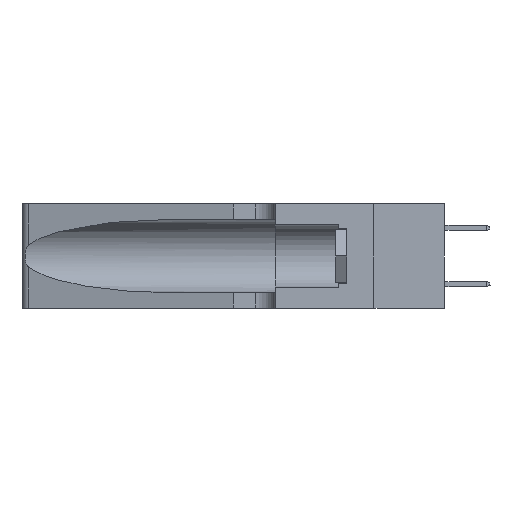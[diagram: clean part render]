
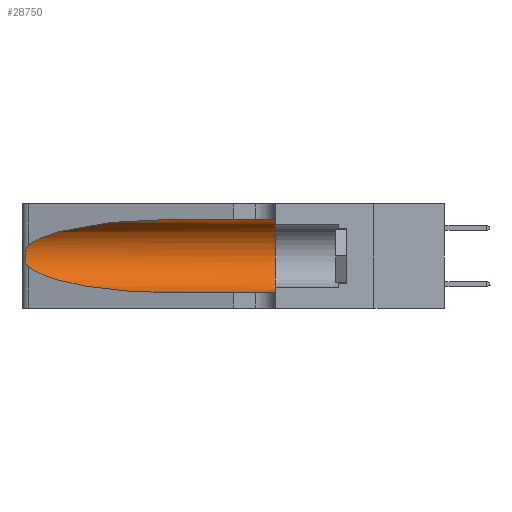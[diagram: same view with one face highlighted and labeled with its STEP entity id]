
A CAD part, left-side view. The second image highlights one B-rep face of the part: STEP entity #28750.
In plain terms, the highlighted cylindrical face has radius 3.308 mm (diameter 6.617 mm), a partial arc.
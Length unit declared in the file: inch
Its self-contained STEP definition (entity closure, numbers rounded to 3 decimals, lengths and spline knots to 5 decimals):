
#1420 = CARTESIAN_POINT ( 'NONE',  ( 0.1305, 0.72297, 0.05475 ) ) ;
#2338 = EDGE_CURVE ( 'NONE', #28870, #16854, #35391, .T. ) ;
#2971 = CARTESIAN_POINT ( 'NONE',  ( 0.25487, 1.22718, 0.14631 ) ) ;
#4224 = EDGE_CURVE ( 'NONE', #25552, #4674, #34730, .T. ) ;
#4225 = AXIS2_PLACEMENT_3D ( 'NONE', #11560, #11099, #27689 ) ;
#4227 = DIRECTION ( 'NONE',  ( 0., 1., 0. ) ) ;
#4668 = ORIENTED_EDGE ( 'NONE', *, *, #24497, .F. ) ;
#4674 = VERTEX_POINT ( 'NONE', #14045 ) ;
#5128 = CARTESIAN_POINT ( 'NONE',  ( 0.1305, 0.72297, 0.05475 ) ) ;
#5406 = EDGE_CURVE ( 'NONE', #4674, #28870, #21373, .T. ) ;
#5975 = CARTESIAN_POINT ( 'NONE',  ( 0.25639, 1.23184, 0.21858 ) ) ;
#7734 = CARTESIAN_POINT ( 'NONE',  ( 0.25487, 1.22718, 0.14631 ) ) ;
#9146 = CARTESIAN_POINT ( 'NONE',  ( 0.25639, 1.23186, 0.15144 ) ) ;
#9158 = EDGE_LOOP ( 'NONE', ( #30131, #21427, #10107, #10745, #4668, #17406 ) ) ;
#9277 = CARTESIAN_POINT ( 'NONE',  ( 0.25854, 1.2359, 0.20912 ) ) ;
#9411 = CARTESIAN_POINT ( 'NONE',  ( 0.25555, 1.22993, 0.14849 ) ) ;
#10107 = ORIENTED_EDGE ( 'NONE', *, *, #5406, .T. ) ;
#10640 = CARTESIAN_POINT ( 'NONE',  ( 0.1305, 0.72297, 0.31525 ) ) ;
#10745 = ORIENTED_EDGE ( 'NONE', *, *, #2338, .T. ) ;
#11099 = DIRECTION ( 'NONE',  ( 0., -1., 0. ) ) ;
#11136 = EDGE_CURVE ( 'NONE', #39856, #25552, #27072, .T. ) ;
#11274 = CARTESIAN_POINT ( 'NONE',  ( 0.2373, 1.15595, 0.28018 ) ) ;
#11437 = VERTEX_POINT ( 'NONE', #25014 ) ;
#11560 = CARTESIAN_POINT ( 'NONE',  ( 0.1305, 1.61858, 0.185 ) ) ;
#11943 = CARTESIAN_POINT ( 'NONE',  ( 0.1305, 0.35, 0.05475 ) ) ;
#12255 = CARTESIAN_POINT ( 'NONE',  ( 0.25787, 1.23484, 0.2124 ) ) ;
#12767 = DIRECTION ( 'NONE',  ( 0., -1., 0. ) ) ;
#14045 = CARTESIAN_POINT ( 'NONE',  ( 0.25487, 1.22718, 0.14631 ) ) ;
#14901 = CARTESIAN_POINT ( 'NONE',  ( 0.25487, 1.22718, 0.22369 ) ) ;
#16854 = VERTEX_POINT ( 'NONE', #11943 ) ;
#17406 = ORIENTED_EDGE ( 'NONE', *, *, #21244, .F. ) ;
#18690 = CARTESIAN_POINT ( 'NONE',  ( 0.25856, 1.23593, 0.16098 ) ) ;
#19502 = VECTOR ( 'NONE', #21400, 39.37008 ) ;
#20017 = CIRCLE ( 'NONE', #24137, 0.13025 ) ;
#20641 = DIRECTION ( 'NONE',  ( 0., 0., 1. ) ) ;
#21244 = EDGE_CURVE ( 'NONE', #39856, #11437, #21584, .T. ) ;
#21373 =( BOUNDED_CURVE ( )  B_SPLINE_CURVE ( 3, ( #7734, #23557, #28028, #1420 ),
 .UNSPECIFIED., .F., .F. ) 
 B_SPLINE_CURVE_WITH_KNOTS ( ( 4, 4 ),
 ( 3.44316, 4.71239 ),
 .UNSPECIFIED. ) 
 CURVE ( )  GEOMETRIC_REPRESENTATION_ITEM ( )  RATIONAL_B_SPLINE_CURVE ( ( 1., 0.87, 0.87, 1. ) ) 
 REPRESENTATION_ITEM ( '' )  );
#21400 = DIRECTION ( 'NONE',  ( 0., -1., 0. ) ) ;
#21427 = ORIENTED_EDGE ( 'NONE', *, *, #4224, .T. ) ;
#21584 = LINE ( 'NONE', #27388, #19502 ) ;
#22190 = FACE_OUTER_BOUND ( 'NONE', #9158, .T. ) ;
#22271 = CARTESIAN_POINT ( 'NONE',  ( 0.25789, 1.23486, 0.15765 ) ) ;
#22523 = CARTESIAN_POINT ( 'NONE',  ( 0.26017, 1.23833, 0.17102 ) ) ;
#23557 = CARTESIAN_POINT ( 'NONE',  ( 0.2373, 1.15595, 0.08982 ) ) ;
#24137 = AXIS2_PLACEMENT_3D ( 'NONE', #40005, #4227, #20641 ) ;
#24497 = EDGE_CURVE ( 'NONE', #11437, #16854, #20017, .T. ) ;
#25014 = CARTESIAN_POINT ( 'NONE',  ( 0.1305, 0.35, 0.31525 ) ) ;
#25552 = VERTEX_POINT ( 'NONE', #14901 ) ;
#27072 =( BOUNDED_CURVE ( )  B_SPLINE_CURVE ( 3, ( #41065, #27386, #11274, #40479 ),
 .UNSPECIFIED., .F., .T. ) 
 B_SPLINE_CURVE_WITH_KNOTS ( ( 4, 4 ),
 ( 1.5708, 2.84003 ),
 .UNSPECIFIED. ) 
 CURVE ( )  GEOMETRIC_REPRESENTATION_ITEM ( )  RATIONAL_B_SPLINE_CURVE ( ( 1., 0.87, 0.87, 1. ) ) 
 REPRESENTATION_ITEM ( '' )  );
#27222 = CARTESIAN_POINT ( 'NONE',  ( 0.25487, 1.22718, 0.22369 ) ) ;
#27386 = CARTESIAN_POINT ( 'NONE',  ( 0.18966, 0.96281, 0.31525 ) ) ;
#27388 = CARTESIAN_POINT ( 'NONE',  ( 0.1305, 1.61858, 0.31525 ) ) ;
#27689 = DIRECTION ( 'NONE',  ( 0., 0., -1. ) ) ;
#28028 = CARTESIAN_POINT ( 'NONE',  ( 0.18966, 0.96281, 0.05475 ) ) ;
#28529 = CARTESIAN_POINT ( 'NONE',  ( 0.26018, 1.23835, 0.19895 ) ) ;
#28750 = ADVANCED_FACE ( 'NONE', ( #22190 ), #29772, .F. ) ;
#28870 = VERTEX_POINT ( 'NONE', #5128 ) ;
#29152 = CARTESIAN_POINT ( 'NONE',  ( 0.1305, 1.61858, 0.05475 ) ) ;
#29772 = CYLINDRICAL_SURFACE ( 'NONE', #4225, 0.13025 ) ;
#30131 = ORIENTED_EDGE ( 'NONE', *, *, #11136, .T. ) ;
#31785 = VECTOR ( 'NONE', #12767, 39.37008 ) ;
#34730 = B_SPLINE_CURVE_WITH_KNOTS ( 'NONE', 3,
 ( #27222, #42177, #5975, #12255, #9277, #28529, #38746, #38341, #22523, #18690, #22271, #9146, #9411, #2971 ),
 .UNSPECIFIED., .F., .F.,
 ( 4, 2, 2, 2, 2, 2, 4 ),
 ( 0., 0.00027, 0.00053, 0.00107, 0.0016, 0.00187, 0.00214 ),
 .UNSPECIFIED. ) ;
#35391 = LINE ( 'NONE', #29152, #31785 ) ;
#38341 = CARTESIAN_POINT ( 'NONE',  ( 0.26075, 1.23896, 0.178 ) ) ;
#38746 = CARTESIAN_POINT ( 'NONE',  ( 0.26075, 1.23896, 0.19203 ) ) ;
#39856 = VERTEX_POINT ( 'NONE', #10640 ) ;
#40005 = CARTESIAN_POINT ( 'NONE',  ( 0.1305, 0.35, 0.185 ) ) ;
#40479 = CARTESIAN_POINT ( 'NONE',  ( 0.25487, 1.22718, 0.22369 ) ) ;
#41065 = CARTESIAN_POINT ( 'NONE',  ( 0.1305, 0.72297, 0.31525 ) ) ;
#42177 = CARTESIAN_POINT ( 'NONE',  ( 0.25555, 1.22994, 0.2215 ) ) ;
